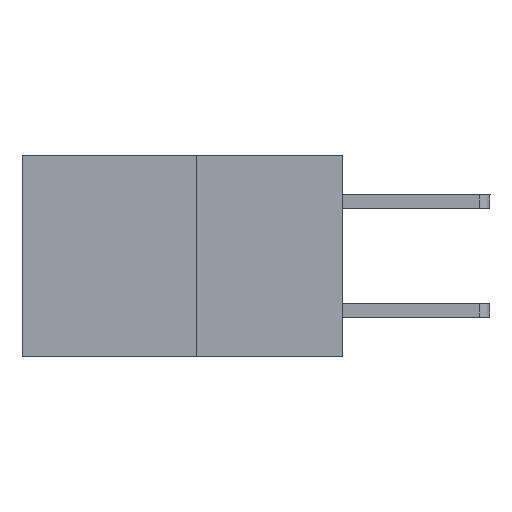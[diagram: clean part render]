
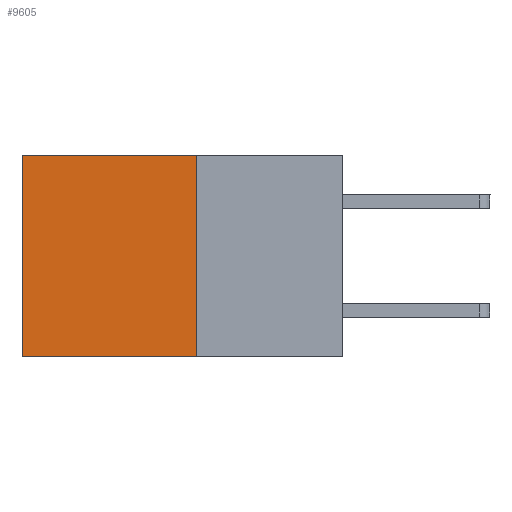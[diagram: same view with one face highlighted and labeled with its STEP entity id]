
A CAD part, left-side view. The second image highlights one B-rep face of the part: STEP entity #9605.
In plain terms, the highlighted planar face has unit normal (-1, 0, 0).
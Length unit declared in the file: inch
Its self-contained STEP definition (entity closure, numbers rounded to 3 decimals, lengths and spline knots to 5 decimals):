
#364 = EDGE_CURVE ( 'NONE', #1962, #7803, #4228, .T. ) ;
#398 = ORIENTED_EDGE ( 'NONE', *, *, #1559, .F. ) ;
#466 = DIRECTION ( 'NONE',  ( 0., 0., -1. ) ) ;
#876 = VECTOR ( 'NONE', #11213, 39.37008 ) ;
#932 = CARTESIAN_POINT ( 'NONE',  ( 0.277, 0.59, 0. ) ) ;
#1382 = CARTESIAN_POINT ( 'NONE',  ( 0.277, 0.27, 0. ) ) ;
#1415 = EDGE_CURVE ( 'NONE', #2661, #5227, #3944, .T. ) ;
#1559 = EDGE_CURVE ( 'NONE', #7803, #5227, #2357, .T. ) ;
#1962 = VERTEX_POINT ( 'NONE', #1382 ) ;
#2357 = LINE ( 'NONE', #5102, #3916 ) ;
#2661 = VERTEX_POINT ( 'NONE', #932 ) ;
#2969 = DIRECTION ( 'NONE',  ( 0., 0., -1. ) ) ;
#3596 = EDGE_LOOP ( 'NONE', ( #10299, #398, #9240, #10076 ) ) ;
#3852 = VECTOR ( 'NONE', #466, 39.37008 ) ;
#3916 = VECTOR ( 'NONE', #10525, 39.37008 ) ;
#3944 = LINE ( 'NONE', #4510, #4692 ) ;
#4228 = LINE ( 'NONE', #5977, #3852 ) ;
#4483 = CARTESIAN_POINT ( 'NONE',  ( 0.277, 0.59, -0.37 ) ) ;
#4510 = CARTESIAN_POINT ( 'NONE',  ( 0.277, 0.59, -0.37 ) ) ;
#4692 = VECTOR ( 'NONE', #2969, 39.37008 ) ;
#4778 = PLANE ( 'NONE',  #10612 ) ;
#5102 = CARTESIAN_POINT ( 'NONE',  ( 0.277, 0.27, -0.37 ) ) ;
#5227 = VERTEX_POINT ( 'NONE', #4483 ) ;
#5616 = DIRECTION ( 'NONE',  ( 0., 0., -1. ) ) ;
#5977 = CARTESIAN_POINT ( 'NONE',  ( 0.277, 0.27, -0.37 ) ) ;
#6537 = DIRECTION ( 'NONE',  ( 1., 0., 0. ) ) ;
#6593 = FACE_OUTER_BOUND ( 'NONE', #3596, .T. ) ;
#7540 = LINE ( 'NONE', #10194, #876 ) ;
#7625 = EDGE_CURVE ( 'NONE', #1962, #2661, #7540, .T. ) ;
#7803 = VERTEX_POINT ( 'NONE', #11881 ) ;
#8273 = CARTESIAN_POINT ( 'NONE',  ( 0.277, 0.27, -0.37 ) ) ;
#9240 = ORIENTED_EDGE ( 'NONE', *, *, #364, .F. ) ;
#9605 = ADVANCED_FACE ( 'NONE', ( #6593 ), #4778, .F. ) ;
#10076 = ORIENTED_EDGE ( 'NONE', *, *, #7625, .T. ) ;
#10194 = CARTESIAN_POINT ( 'NONE',  ( 0.277, 0.27, 0. ) ) ;
#10299 = ORIENTED_EDGE ( 'NONE', *, *, #1415, .T. ) ;
#10525 = DIRECTION ( 'NONE',  ( 0., 1., 0. ) ) ;
#10612 = AXIS2_PLACEMENT_3D ( 'NONE', #8273, #6537, #5616 ) ;
#11213 = DIRECTION ( 'NONE',  ( 0., 1., 0. ) ) ;
#11881 = CARTESIAN_POINT ( 'NONE',  ( 0.277, 0.27, -0.37 ) ) ;
